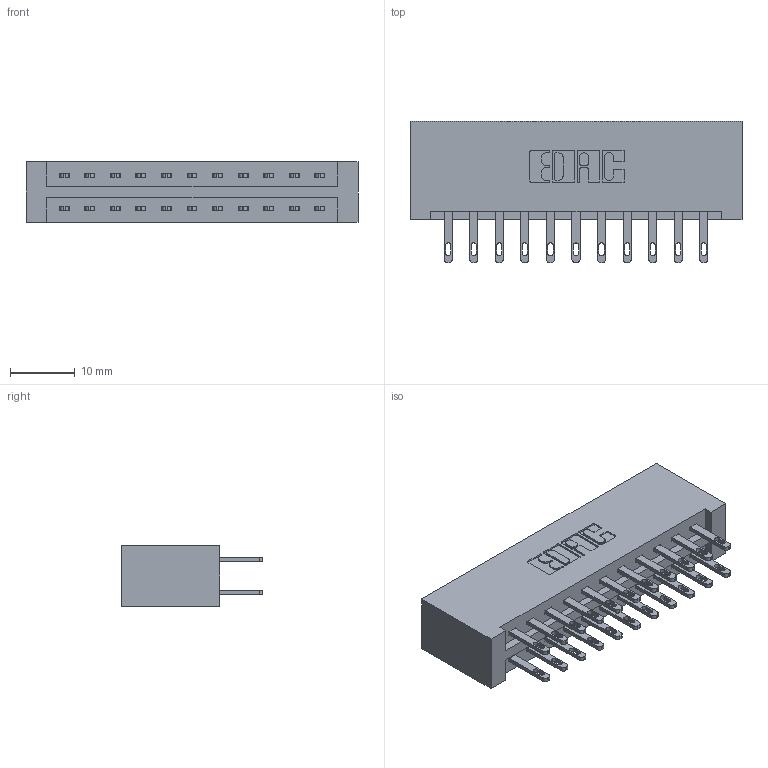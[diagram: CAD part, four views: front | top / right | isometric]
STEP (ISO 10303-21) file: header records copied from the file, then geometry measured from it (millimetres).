
FILE_DESCRIPTION (( 'STEP AP203' ), '1' );
FILE_NAME ('337-022-500-201.STEP', '2018-08-05T12:23:16', ( '' ), ( '' ), 'SwSTEP 2.0', 'SolidWorks 2016', '' );
FILE_SCHEMA (( 'CONFIG_CONTROL_DESIGN' ));
Length unit declared in the file: inch
Products named in the file (3): 337 Part_No Mounting Lugs; 345-292-001_345-293-100; 337-022-500-201
Assembly tree (23 placements, depth 2):
  337-022-500-201
    337 Part_No Mounting Lugs
    345-292-001_345-293-100  x22
Bounding box: 51.46 x 21.85 x 9.4 mm (x, y, z)
Volume: 5838.6 mm3; surface area: 6599.7 mm2
Topology: 23 solids, 23 shells, 1206 faces, 3653 edges, 2434 vertices
Faces by surface type: plane 770, cylinder 436
Entity records: 12191 total; most frequent: CARTESIAN_POINT 2078, ORIENTED_EDGE 2014, DIRECTION 1819, EDGE_CURVE 1007, VECTOR 883, LINE 883, VERTEX_POINT 670, AXIS2_PLACEMENT_3D 468
